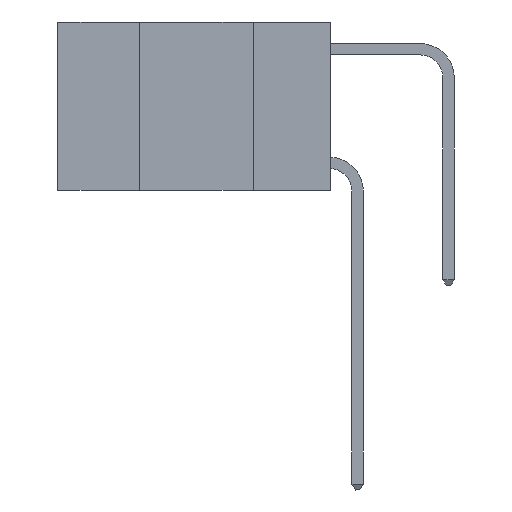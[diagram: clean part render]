
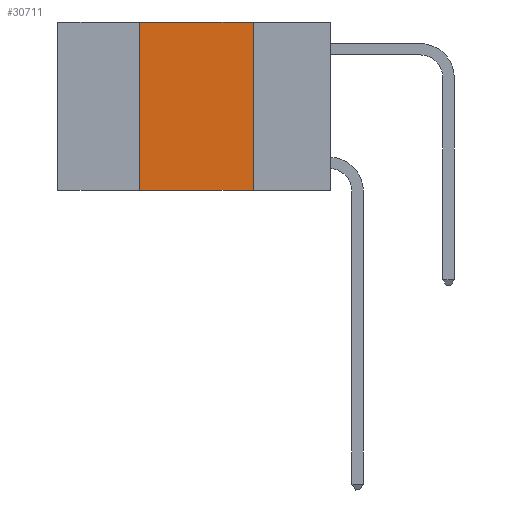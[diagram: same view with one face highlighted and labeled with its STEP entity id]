
A CAD part, left-side view. The second image highlights one B-rep face of the part: STEP entity #30711.
In plain terms, the highlighted planar face has unit normal (-1, 0, 0).
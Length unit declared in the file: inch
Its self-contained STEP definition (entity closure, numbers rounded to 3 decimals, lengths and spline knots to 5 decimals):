
#38 = DIRECTION ( 'NONE',  ( 0., 0., -1. ) ) ;
#750 = VERTEX_POINT ( 'NONE', #5138 ) ;
#1721 = CARTESIAN_POINT ( 'NONE',  ( 0., 0.17, 0. ) ) ;
#1975 = LINE ( 'NONE', #9791, #6062 ) ;
#2387 = CARTESIAN_POINT ( 'NONE',  ( 0., 0.6, 0. ) ) ;
#2446 = DIRECTION ( 'NONE',  ( 0., -1., 0. ) ) ;
#4053 = DIRECTION ( 'NONE',  ( 0., -1., 0. ) ) ;
#5138 = CARTESIAN_POINT ( 'NONE',  ( 0., 0.17, -0.37 ) ) ;
#6062 = VECTOR ( 'NONE', #19626, 39.37008 ) ;
#6531 = EDGE_LOOP ( 'NONE', ( #15390, #30624, #18998, #6910 ) ) ;
#6910 = ORIENTED_EDGE ( 'NONE', *, *, #25264, .T. ) ;
#9716 = CARTESIAN_POINT ( 'NONE',  ( 0., 0.17, 0. ) ) ;
#9791 = CARTESIAN_POINT ( 'NONE',  ( 0., 0.42, 0. ) ) ;
#10535 = VECTOR ( 'NONE', #29581, 39.37008 ) ;
#13035 = DIRECTION ( 'NONE',  ( 1., 0., 0. ) ) ;
#14688 = EDGE_CURVE ( 'NONE', #25944, #27884, #1975, .T. ) ;
#15390 = ORIENTED_EDGE ( 'NONE', *, *, #22804, .F. ) ;
#16714 = CARTESIAN_POINT ( 'NONE',  ( 0., 0.6, -0.37 ) ) ;
#17271 = LINE ( 'NONE', #22754, #25685 ) ;
#18998 = ORIENTED_EDGE ( 'NONE', *, *, #14688, .F. ) ;
#19536 = LINE ( 'NONE', #16714, #23411 ) ;
#19626 = DIRECTION ( 'NONE',  ( 0., 0., 1. ) ) ;
#22336 = EDGE_CURVE ( 'NONE', #27884, #25283, #17271, .T. ) ;
#22754 = CARTESIAN_POINT ( 'NONE',  ( 0., 0.6, 0. ) ) ;
#22804 = EDGE_CURVE ( 'NONE', #25283, #750, #32234, .T. ) ;
#23411 = VECTOR ( 'NONE', #4053, 39.37008 ) ;
#25264 = EDGE_CURVE ( 'NONE', #25944, #750, #19536, .T. ) ;
#25283 = VERTEX_POINT ( 'NONE', #1721 ) ;
#25685 = VECTOR ( 'NONE', #2446, 39.37008 ) ;
#25713 = FACE_OUTER_BOUND ( 'NONE', #6531, .T. ) ;
#25944 = VERTEX_POINT ( 'NONE', #31322 ) ;
#26729 = CARTESIAN_POINT ( 'NONE',  ( 0., 0.42, 0. ) ) ;
#27884 = VERTEX_POINT ( 'NONE', #26729 ) ;
#29581 = DIRECTION ( 'NONE',  ( 0., 0., -1. ) ) ;
#30220 = PLANE ( 'NONE',  #30413 ) ;
#30413 = AXIS2_PLACEMENT_3D ( 'NONE', #2387, #13035, #38 ) ;
#30624 = ORIENTED_EDGE ( 'NONE', *, *, #22336, .F. ) ;
#30711 = ADVANCED_FACE ( 'NONE', ( #25713 ), #30220, .F. ) ;
#31322 = CARTESIAN_POINT ( 'NONE',  ( 0., 0.42, -0.37 ) ) ;
#32234 = LINE ( 'NONE', #9716, #10535 ) ;
